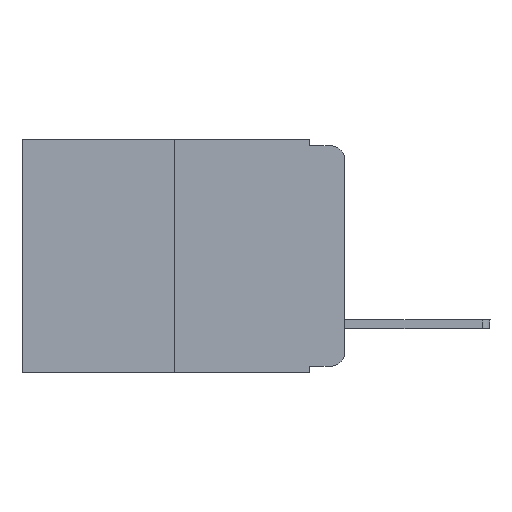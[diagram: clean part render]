
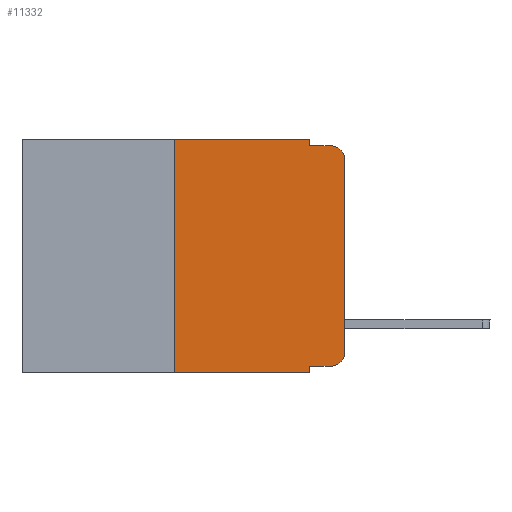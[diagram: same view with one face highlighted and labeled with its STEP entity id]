
A CAD part, left-side view. The second image highlights one B-rep face of the part: STEP entity #11332.
In plain terms, the highlighted planar face has unit normal (-1, 0, 0).
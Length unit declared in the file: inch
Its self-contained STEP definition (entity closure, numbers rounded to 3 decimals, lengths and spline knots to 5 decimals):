
#261 = CARTESIAN_POINT ( 'NONE',  ( 0., 0.02, -0.01 ) ) ;
#444 = VERTEX_POINT ( 'NONE', #9906 ) ;
#1026 = VECTOR ( 'NONE', #9250, 39.37008 ) ;
#1449 = CARTESIAN_POINT ( 'NONE',  ( 0., 0.473, 0. ) ) ;
#1487 = DIRECTION ( 'NONE',  ( -1., 0., 0. ) ) ;
#2937 = ORIENTED_EDGE ( 'NONE', *, *, #9195, .F. ) ;
#2995 = AXIS2_PLACEMENT_3D ( 'NONE', #17269, #17141, #9809 ) ;
#3079 = ORIENTED_EDGE ( 'NONE', *, *, #3354, .T. ) ;
#3177 = CARTESIAN_POINT ( 'NONE',  ( 0., 0.051, -0.01 ) ) ;
#3354 = EDGE_CURVE ( 'NONE', #14554, #12013, #14335, .T. ) ;
#3739 = ORIENTED_EDGE ( 'NONE', *, *, #15718, .T. ) ;
#3988 = LINE ( 'NONE', #1449, #13696 ) ;
#4968 = DIRECTION ( 'NONE',  ( 1., 0., 0. ) ) ;
#5158 = CARTESIAN_POINT ( 'NONE',  ( 0., 0.02, -0.03 ) ) ;
#5306 = DIRECTION ( 'NONE',  ( 0., 0., -1. ) ) ;
#5886 = VERTEX_POINT ( 'NONE', #15590 ) ;
#6193 = VECTOR ( 'NONE', #13188, 39.37008 ) ;
#6465 = CARTESIAN_POINT ( 'NONE',  ( 0., 0., 0. ) ) ;
#6676 = EDGE_CURVE ( 'NONE', #5886, #18186, #14757, .T. ) ;
#7302 = CARTESIAN_POINT ( 'NONE',  ( 0., 0.051, -0.343 ) ) ;
#7332 = EDGE_CURVE ( 'NONE', #444, #14554, #15917, .T. ) ;
#8130 = ORIENTED_EDGE ( 'NONE', *, *, #17990, .F. ) ;
#8575 = VERTEX_POINT ( 'NONE', #20841 ) ;
#8677 = FACE_OUTER_BOUND ( 'NONE', #9323, .T. ) ;
#8833 = EDGE_CURVE ( 'NONE', #18186, #20680, #3988, .T. ) ;
#8846 = ORIENTED_EDGE ( 'NONE', *, *, #8833, .F. ) ;
#8990 = DIRECTION ( 'NONE',  ( 0., 0., -1. ) ) ;
#9195 = EDGE_CURVE ( 'NONE', #20680, #8575, #19807, .T. ) ;
#9250 = DIRECTION ( 'NONE',  ( 0., 0., 1. ) ) ;
#9323 = EDGE_LOOP ( 'NONE', ( #11346, #14284, #22348, #2937, #8846, #12935, #3739, #8130, #17578, #3079 ) ) ;
#9499 = CARTESIAN_POINT ( 'NONE',  ( 0., 0.25, 0. ) ) ;
#9645 = EDGE_CURVE ( 'NONE', #20552, #13195, #20345, .T. ) ;
#9656 = DIRECTION ( 'NONE',  ( 0., -1., 0. ) ) ;
#9705 = CARTESIAN_POINT ( 'NONE',  ( 0., 0., -0.313 ) ) ;
#9809 = DIRECTION ( 'NONE',  ( 0., 0., -1. ) ) ;
#9906 = CARTESIAN_POINT ( 'NONE',  ( 0., 0.051, -0.333 ) ) ;
#10684 = DIRECTION ( 'NONE',  ( 0., -1., 0. ) ) ;
#10838 = VECTOR ( 'NONE', #10684, 39.37008 ) ;
#11257 = VECTOR ( 'NONE', #19709, 39.37008 ) ;
#11332 = ADVANCED_FACE ( 'NONE', ( #8677 ), #23606, .F. ) ;
#11346 = ORIENTED_EDGE ( 'NONE', *, *, #17308, .T. ) ;
#11939 = CARTESIAN_POINT ( 'NONE',  ( 0., 0.02, -0.333 ) ) ;
#12013 = VERTEX_POINT ( 'NONE', #9705 ) ;
#12016 = CARTESIAN_POINT ( 'NONE',  ( 0., 0.051, 0. ) ) ;
#12646 = LINE ( 'NONE', #3177, #10838 ) ;
#12935 = ORIENTED_EDGE ( 'NONE', *, *, #6676, .F. ) ;
#13188 = DIRECTION ( 'NONE',  ( 0., -1., 0. ) ) ;
#13195 = VERTEX_POINT ( 'NONE', #261 ) ;
#13380 = CARTESIAN_POINT ( 'NONE',  ( 0., 0.051, 0. ) ) ;
#13696 = VECTOR ( 'NONE', #9656, 39.37008 ) ;
#13875 = CARTESIAN_POINT ( 'NONE',  ( 0., 0.25, 0. ) ) ;
#14211 = CARTESIAN_POINT ( 'NONE',  ( 0., 0.473, -0.343 ) ) ;
#14284 = ORIENTED_EDGE ( 'NONE', *, *, #9645, .T. ) ;
#14335 = CIRCLE ( 'NONE', #2995, 0.02 ) ;
#14554 = VERTEX_POINT ( 'NONE', #11939 ) ;
#14757 = LINE ( 'NONE', #9499, #1026 ) ;
#15423 = CARTESIAN_POINT ( 'NONE',  ( 0., 0., -0.03 ) ) ;
#15590 = CARTESIAN_POINT ( 'NONE',  ( 0., 0.25, -0.343 ) ) ;
#15718 = EDGE_CURVE ( 'NONE', #5886, #18754, #20078, .T. ) ;
#15917 = LINE ( 'NONE', #23384, #22972 ) ;
#16351 = VECTOR ( 'NONE', #22537, 39.37008 ) ;
#17141 = DIRECTION ( 'NONE',  ( -1., 0., 0. ) ) ;
#17269 = CARTESIAN_POINT ( 'NONE',  ( 0., 0.02, -0.313 ) ) ;
#17308 = EDGE_CURVE ( 'NONE', #12013, #20552, #23378, .T. ) ;
#17578 = ORIENTED_EDGE ( 'NONE', *, *, #7332, .T. ) ;
#17990 = EDGE_CURVE ( 'NONE', #444, #18754, #20593, .T. ) ;
#18018 = AXIS2_PLACEMENT_3D ( 'NONE', #5158, #1487, #8990 ) ;
#18186 = VERTEX_POINT ( 'NONE', #13875 ) ;
#18754 = VERTEX_POINT ( 'NONE', #7302 ) ;
#19709 = DIRECTION ( 'NONE',  ( 0., 0., 1. ) ) ;
#19807 = LINE ( 'NONE', #22089, #21516 ) ;
#19947 = DIRECTION ( 'NONE',  ( 0., 0., -1. ) ) ;
#20078 = LINE ( 'NONE', #14211, #6193 ) ;
#20345 = CIRCLE ( 'NONE', #18018, 0.02 ) ;
#20552 = VERTEX_POINT ( 'NONE', #15423 ) ;
#20593 = LINE ( 'NONE', #13380, #16351 ) ;
#20680 = VERTEX_POINT ( 'NONE', #12016 ) ;
#20841 = CARTESIAN_POINT ( 'NONE',  ( 0., 0.051, -0.01 ) ) ;
#21423 = CARTESIAN_POINT ( 'NONE',  ( 0., 0.473, 0. ) ) ;
#21516 = VECTOR ( 'NONE', #5306, 39.37008 ) ;
#22089 = CARTESIAN_POINT ( 'NONE',  ( 0., 0.051, 0. ) ) ;
#22158 = EDGE_CURVE ( 'NONE', #8575, #13195, #12646, .T. ) ;
#22348 = ORIENTED_EDGE ( 'NONE', *, *, #22158, .F. ) ;
#22537 = DIRECTION ( 'NONE',  ( 0., 0., -1. ) ) ;
#22881 = AXIS2_PLACEMENT_3D ( 'NONE', #21423, #4968, #19947 ) ;
#22972 = VECTOR ( 'NONE', #23147, 39.37008 ) ;
#23147 = DIRECTION ( 'NONE',  ( 0., -1., 0. ) ) ;
#23378 = LINE ( 'NONE', #6465, #11257 ) ;
#23384 = CARTESIAN_POINT ( 'NONE',  ( 0., 0.051, -0.333 ) ) ;
#23606 = PLANE ( 'NONE',  #22881 ) ;
